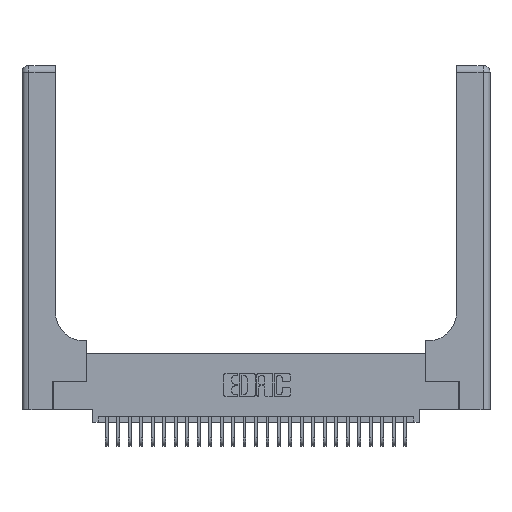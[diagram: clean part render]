
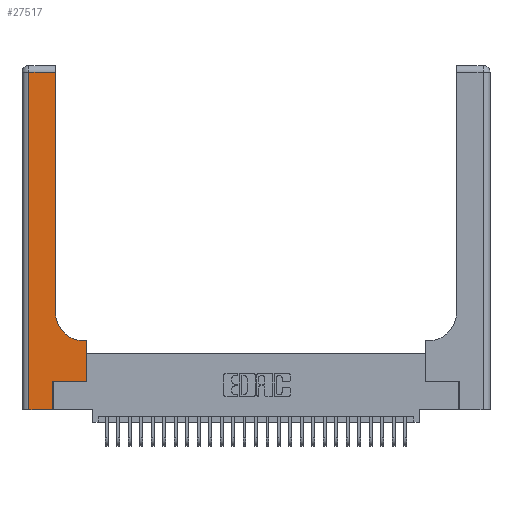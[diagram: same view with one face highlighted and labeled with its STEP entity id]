
A CAD part, top view. The second image highlights one B-rep face of the part: STEP entity #27517.
In plain terms, the highlighted planar face has unit normal (0, 0, 1).
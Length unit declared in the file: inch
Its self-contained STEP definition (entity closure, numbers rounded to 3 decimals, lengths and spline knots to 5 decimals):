
#77 = VERTEX_POINT ( 'NONE', #29716 ) ;
#398 = CARTESIAN_POINT ( 'NONE',  ( 0., 2.94, 0.37 ) ) ;
#841 = DIRECTION ( 'NONE',  ( -1., 0., 0. ) ) ;
#870 = EDGE_CURVE ( 'NONE', #30077, #5529, #27101, .T. ) ;
#1705 = DIRECTION ( 'NONE',  ( 1., 0., 0. ) ) ;
#1771 = EDGE_CURVE ( 'NONE', #77, #15111, #3339, .T. ) ;
#2096 = CARTESIAN_POINT ( 'NONE',  ( 0.06, 2.94, 0.37 ) ) ;
#2247 = ORIENTED_EDGE ( 'NONE', *, *, #16566, .T. ) ;
#2438 = EDGE_CURVE ( 'NONE', #4611, #24076, #11412, .T. ) ;
#3172 = VERTEX_POINT ( 'NONE', #24003 ) ;
#3339 = LINE ( 'NONE', #398, #27385 ) ;
#3621 = VERTEX_POINT ( 'NONE', #4402 ) ;
#4005 = VECTOR ( 'NONE', #21915, 39.37008 ) ;
#4289 = EDGE_CURVE ( 'NONE', #27720, #3621, #29311, .T. ) ;
#4402 = CARTESIAN_POINT ( 'NONE',  ( 0.269, 0., 0.37 ) ) ;
#4611 = VERTEX_POINT ( 'NONE', #14734 ) ;
#5167 = VECTOR ( 'NONE', #5397, 39.37008 ) ;
#5397 = DIRECTION ( 'NONE',  ( 1., 0., 0. ) ) ;
#5529 = VERTEX_POINT ( 'NONE', #9050 ) ;
#5687 = CARTESIAN_POINT ( 'NONE',  ( 0.2915, 3., 0.37 ) ) ;
#5821 = ORIENTED_EDGE ( 'NONE', *, *, #4289, .T. ) ;
#6961 = PLANE ( 'NONE',  #8449 ) ;
#7409 = FACE_OUTER_BOUND ( 'NONE', #8943, .T. ) ;
#8449 = AXIS2_PLACEMENT_3D ( 'NONE', #13857, #23154, #9305 ) ;
#8943 = EDGE_LOOP ( 'NONE', ( #19781, #24317, #22561, #5821, #2247, #28221, #23726, #29965, #17862 ) ) ;
#9050 = CARTESIAN_POINT ( 'NONE',  ( 0.2915, 0.85, 0.37 ) ) ;
#9305 = DIRECTION ( 'NONE',  ( -1., 0., 0. ) ) ;
#10425 = VECTOR ( 'NONE', #25044, 39.37008 ) ;
#11262 = CARTESIAN_POINT ( 'NONE',  ( 0.5415, 0.6, 0.37 ) ) ;
#11387 = EDGE_CURVE ( 'NONE', #5529, #77, #27995, .T. ) ;
#11412 = LINE ( 'NONE', #28521, #5167 ) ;
#13484 = CARTESIAN_POINT ( 'NONE',  ( 0.269, 0., 0.37 ) ) ;
#13760 = VECTOR ( 'NONE', #15792, 39.37008 ) ;
#13857 = CARTESIAN_POINT ( 'NONE',  ( 0., 3., 0.37 ) ) ;
#14313 = CARTESIAN_POINT ( 'NONE',  ( 0.06, 3., 0.37 ) ) ;
#14535 = CARTESIAN_POINT ( 'NONE',  ( 0.06, 0., 0.37 ) ) ;
#14734 = CARTESIAN_POINT ( 'NONE',  ( 0.269, 0.25, 0.37 ) ) ;
#15111 = VERTEX_POINT ( 'NONE', #2096 ) ;
#15737 = DIRECTION ( 'NONE',  ( 0., 0., -1. ) ) ;
#15792 = DIRECTION ( 'NONE',  ( 0., 1., 0. ) ) ;
#16535 = LINE ( 'NONE', #18043, #10425 ) ;
#16566 = EDGE_CURVE ( 'NONE', #3621, #4611, #19917, .T. ) ;
#16885 = DIRECTION ( 'NONE',  ( -1., 0., 0. ) ) ;
#16969 = LINE ( 'NONE', #14313, #28597 ) ;
#17207 = CARTESIAN_POINT ( 'NONE',  ( 0.2915, 0.6, 0.37 ) ) ;
#17845 = EDGE_CURVE ( 'NONE', #24076, #3172, #16535, .T. ) ;
#17862 = ORIENTED_EDGE ( 'NONE', *, *, #870, .T. ) ;
#18043 = CARTESIAN_POINT ( 'NONE',  ( 0.5585, 0.25, 0.37 ) ) ;
#19781 = ORIENTED_EDGE ( 'NONE', *, *, #11387, .T. ) ;
#19917 = LINE ( 'NONE', #13484, #13760 ) ;
#20505 = EDGE_CURVE ( 'NONE', #3172, #30077, #27341, .T. ) ;
#21159 = VECTOR ( 'NONE', #841, 39.37008 ) ;
#21915 = DIRECTION ( 'NONE',  ( 0., 1., 0. ) ) ;
#22561 = ORIENTED_EDGE ( 'NONE', *, *, #24862, .T. ) ;
#22879 = CARTESIAN_POINT ( 'NONE',  ( 0.5585, 0.25, 0.37 ) ) ;
#22962 = CARTESIAN_POINT ( 'NONE',  ( 0., 0., 0.37 ) ) ;
#23151 = VECTOR ( 'NONE', #27635, 39.37008 ) ;
#23154 = DIRECTION ( 'NONE',  ( 0., 0., -1. ) ) ;
#23726 = ORIENTED_EDGE ( 'NONE', *, *, #17845, .T. ) ;
#24003 = CARTESIAN_POINT ( 'NONE',  ( 0.5585, 0.6, 0.37 ) ) ;
#24076 = VERTEX_POINT ( 'NONE', #22879 ) ;
#24317 = ORIENTED_EDGE ( 'NONE', *, *, #1771, .T. ) ;
#24862 = EDGE_CURVE ( 'NONE', #15111, #27720, #16969, .T. ) ;
#25044 = DIRECTION ( 'NONE',  ( 0., 1., 0. ) ) ;
#25083 = AXIS2_PLACEMENT_3D ( 'NONE', #29609, #15737, #1705 ) ;
#25847 = DIRECTION ( 'NONE',  ( 0., -1., 0. ) ) ;
#27101 = CIRCLE ( 'NONE', #25083, 0.25 ) ;
#27341 = LINE ( 'NONE', #17207, #21159 ) ;
#27385 = VECTOR ( 'NONE', #16885, 39.37008 ) ;
#27517 = ADVANCED_FACE ( 'NONE', ( #7409 ), #6961, .F. ) ;
#27635 = DIRECTION ( 'NONE',  ( 1., 0., 0. ) ) ;
#27720 = VERTEX_POINT ( 'NONE', #14535 ) ;
#27995 = LINE ( 'NONE', #5687, #4005 ) ;
#28221 = ORIENTED_EDGE ( 'NONE', *, *, #2438, .T. ) ;
#28521 = CARTESIAN_POINT ( 'NONE',  ( 0.269, 0.25, 0.37 ) ) ;
#28597 = VECTOR ( 'NONE', #25847, 39.37008 ) ;
#29311 = LINE ( 'NONE', #22962, #23151 ) ;
#29609 = CARTESIAN_POINT ( 'NONE',  ( 0.5415, 0.85, 0.37 ) ) ;
#29716 = CARTESIAN_POINT ( 'NONE',  ( 0.2915, 2.94, 0.37 ) ) ;
#29965 = ORIENTED_EDGE ( 'NONE', *, *, #20505, .T. ) ;
#30077 = VERTEX_POINT ( 'NONE', #11262 ) ;
